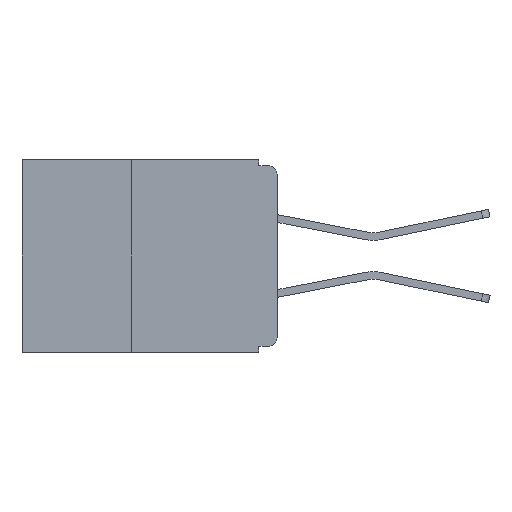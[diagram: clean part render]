
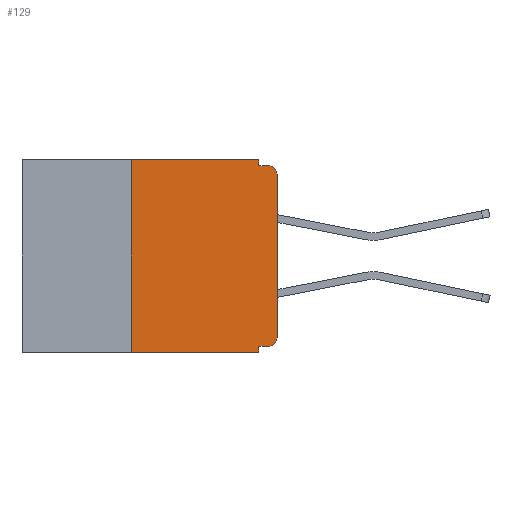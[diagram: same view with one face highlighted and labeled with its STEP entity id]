
A CAD part, left-side view. The second image highlights one B-rep face of the part: STEP entity #129.
In plain terms, the highlighted planar face has unit normal (-1, 0, 0).
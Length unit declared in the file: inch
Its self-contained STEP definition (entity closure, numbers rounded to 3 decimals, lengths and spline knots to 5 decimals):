
#129 = ADVANCED_FACE ( 'NONE', ( #4572 ), #7474, .F. ) ;
#419 = CARTESIAN_POINT ( 'NONE',  ( 0., 0.031, -0.32 ) ) ;
#1270 = VERTEX_POINT ( 'NONE', #5713 ) ;
#1492 = CARTESIAN_POINT ( 'NONE',  ( 0., 0.25, -0.33 ) ) ;
#1493 = VECTOR ( 'NONE', #1603, 39.37008 ) ;
#1571 = LINE ( 'NONE', #1492, #1493 ) ;
#1603 = DIRECTION ( 'NONE',  ( 0., 0., 1. ) ) ;
#2103 = VECTOR ( 'NONE', #6458, 39.37008 ) ;
#2148 = VECTOR ( 'NONE', #6368, 39.37008 ) ;
#2178 = LINE ( 'NONE', #6293, #2103 ) ;
#2261 = LINE ( 'NONE', #6611, #2148 ) ;
#2436 = EDGE_LOOP ( 'NONE', ( #5733, #5881, #6185, #6657, #6956, #7416, #8414, #8564, #8857, #8981 ) ) ;
#2486 = CARTESIAN_POINT ( 'NONE',  ( 0., 0., -0.025 ) ) ;
#2624 = VECTOR ( 'NONE', #8589, 39.37008 ) ;
#2656 = LINE ( 'NONE', #8641, #2624 ) ;
#3413 = VECTOR ( 'NONE', #11976, 39.37008 ) ;
#3434 = DIRECTION ( 'NONE',  ( 0., 0., -1. ) ) ;
#3462 = LINE ( 'NONE', #12004, #3413 ) ;
#3469 = DIRECTION ( 'NONE',  ( -1., 0., 0. ) ) ;
#3559 = CARTESIAN_POINT ( 'NONE',  ( 0., 0.015, -0.305 ) ) ;
#3605 = CARTESIAN_POINT ( 'NONE',  ( 0., 0.25, -0.33 ) ) ;
#3908 = VERTEX_POINT ( 'NONE', #4710 ) ;
#4384 = CARTESIAN_POINT ( 'NONE',  ( 0., 0.015, -0.32 ) ) ;
#4447 = CARTESIAN_POINT ( 'NONE',  ( 0., 0., -0.305 ) ) ;
#4474 = VECTOR ( 'NONE', #10031, 39.37008 ) ;
#4525 = DIRECTION ( 'NONE',  ( 0., 0., -1. ) ) ;
#4548 = VERTEX_POINT ( 'NONE', #4892 ) ;
#4569 = LINE ( 'NONE', #9866, #4474 ) ;
#4572 = FACE_OUTER_BOUND ( 'NONE', #2436, .T. ) ;
#4586 = CARTESIAN_POINT ( 'NONE',  ( 0., 0.031, 0. ) ) ;
#4710 = CARTESIAN_POINT ( 'NONE',  ( 0., 0.031, -0.33 ) ) ;
#4833 = LINE ( 'NONE', #11473, #4874 ) ;
#4874 = VECTOR ( 'NONE', #11554, 39.37008 ) ;
#4892 = CARTESIAN_POINT ( 'NONE',  ( 0., 0.031, -0.01 ) ) ;
#5172 = EDGE_CURVE ( 'NONE', #7447, #9825, #9793, .T. ) ;
#5178 = DIRECTION ( 'NONE',  ( -1., 0., 0. ) ) ;
#5201 = CARTESIAN_POINT ( 'NONE',  ( 0., 0.015, -0.025 ) ) ;
#5384 = VERTEX_POINT ( 'NONE', #2486 ) ;
#5499 = VERTEX_POINT ( 'NONE', #4586 ) ;
#5713 = CARTESIAN_POINT ( 'NONE',  ( 0., 0.25, 0. ) ) ;
#5733 = ORIENTED_EDGE ( 'NONE', *, *, #7236, .T. ) ;
#5881 = ORIENTED_EDGE ( 'NONE', *, *, #11878, .T. ) ;
#5891 = VERTEX_POINT ( 'NONE', #3605 ) ;
#6010 = VECTOR ( 'NONE', #9375, 39.37008 ) ;
#6100 = LINE ( 'NONE', #12120, #6010 ) ;
#6185 = ORIENTED_EDGE ( 'NONE', *, *, #7329, .F. ) ;
#6293 = CARTESIAN_POINT ( 'NONE',  ( 0., 0.031, 0. ) ) ;
#6368 = DIRECTION ( 'NONE',  ( 0., -1., 0. ) ) ;
#6458 = DIRECTION ( 'NONE',  ( 0., 0., -1. ) ) ;
#6611 = CARTESIAN_POINT ( 'NONE',  ( 0., 0., -0.01 ) ) ;
#6657 = ORIENTED_EDGE ( 'NONE', *, *, #7346, .F. ) ;
#6956 = ORIENTED_EDGE ( 'NONE', *, *, #7084, .F. ) ;
#7084 = EDGE_CURVE ( 'NONE', #1270, #5499, #3462, .T. ) ;
#7236 = EDGE_CURVE ( 'NONE', #9825, #5384, #2656, .T. ) ;
#7329 = EDGE_CURVE ( 'NONE', #4548, #8006, #2261, .T. ) ;
#7346 = EDGE_CURVE ( 'NONE', #5499, #4548, #2178, .T. ) ;
#7397 = CARTESIAN_POINT ( 'NONE',  ( 0., 0.437, 0. ) ) ;
#7416 = ORIENTED_EDGE ( 'NONE', *, *, #7557, .F. ) ;
#7447 = VERTEX_POINT ( 'NONE', #4384 ) ;
#7474 = PLANE ( 'NONE',  #11881 ) ;
#7557 = EDGE_CURVE ( 'NONE', #5891, #1270, #1571, .T. ) ;
#8006 = VERTEX_POINT ( 'NONE', #11714 ) ;
#8414 = ORIENTED_EDGE ( 'NONE', *, *, #9644, .T. ) ;
#8468 = CIRCLE ( 'NONE', #11790, 0.015 ) ;
#8564 = ORIENTED_EDGE ( 'NONE', *, *, #10239, .F. ) ;
#8589 = DIRECTION ( 'NONE',  ( 0., 0., 1. ) ) ;
#8641 = CARTESIAN_POINT ( 'NONE',  ( 0., 0., 0. ) ) ;
#8857 = ORIENTED_EDGE ( 'NONE', *, *, #10118, .F. ) ;
#8981 = ORIENTED_EDGE ( 'NONE', *, *, #5172, .T. ) ;
#9375 = DIRECTION ( 'NONE',  ( 0., -1., 0. ) ) ;
#9388 = VERTEX_POINT ( 'NONE', #419 ) ;
#9554 = AXIS2_PLACEMENT_3D ( 'NONE', #3559, #3469, #3434 ) ;
#9644 = EDGE_CURVE ( 'NONE', #5891, #3908, #6100, .T. ) ;
#9793 = CIRCLE ( 'NONE', #9554, 0.015 ) ;
#9825 = VERTEX_POINT ( 'NONE', #4447 ) ;
#9866 = CARTESIAN_POINT ( 'NONE',  ( 0., 0.031, -0.33 ) ) ;
#10031 = DIRECTION ( 'NONE',  ( 0., 0., -1. ) ) ;
#10118 = EDGE_CURVE ( 'NONE', #7447, #9388, #4833, .T. ) ;
#10239 = EDGE_CURVE ( 'NONE', #9388, #3908, #4569, .T. ) ;
#11203 = DIRECTION ( 'NONE',  ( 0., 0., -1. ) ) ;
#11252 = DIRECTION ( 'NONE',  ( 1., 0., 0. ) ) ;
#11473 = CARTESIAN_POINT ( 'NONE',  ( 0., 0., -0.32 ) ) ;
#11554 = DIRECTION ( 'NONE',  ( 0., 1., 0. ) ) ;
#11714 = CARTESIAN_POINT ( 'NONE',  ( 0., 0.015, -0.01 ) ) ;
#11790 = AXIS2_PLACEMENT_3D ( 'NONE', #5201, #5178, #4525 ) ;
#11878 = EDGE_CURVE ( 'NONE', #5384, #8006, #8468, .T. ) ;
#11881 = AXIS2_PLACEMENT_3D ( 'NONE', #7397, #11252, #11203 ) ;
#11976 = DIRECTION ( 'NONE',  ( 0., -1., 0. ) ) ;
#12004 = CARTESIAN_POINT ( 'NONE',  ( 0., 0.437, 0. ) ) ;
#12120 = CARTESIAN_POINT ( 'NONE',  ( 0., 0.437, -0.33 ) ) ;
